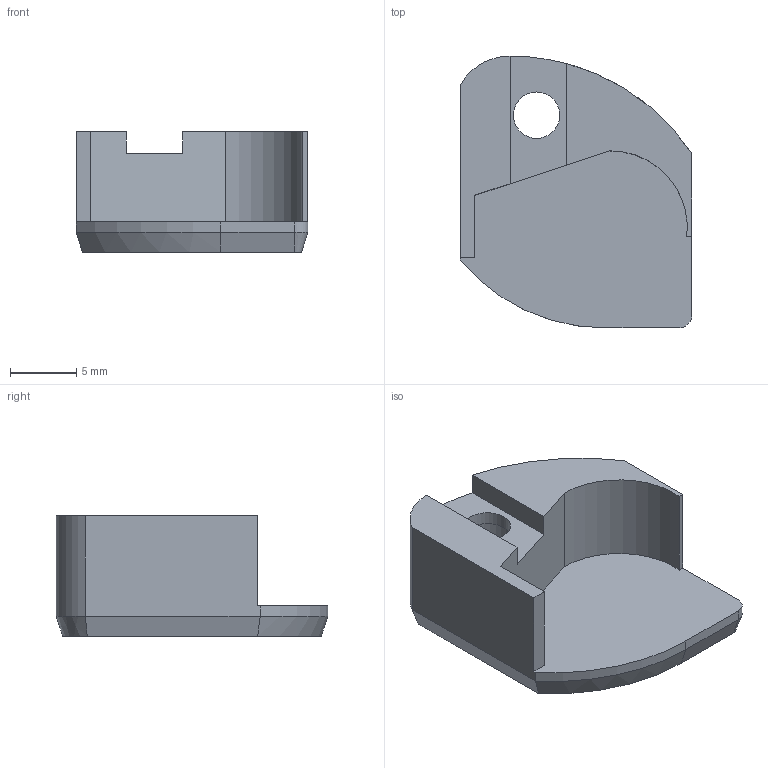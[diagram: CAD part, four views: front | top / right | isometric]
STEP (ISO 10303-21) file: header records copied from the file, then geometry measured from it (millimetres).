
FILE_DESCRIPTION(/* description */ (''),/* implementation_level */ '2;1');
FILE_NAME(/* name */ 'thumb tab side 2 v1.step',/* time_stamp */ '2022-02-13T17:47:28-06:00',/* author */ (''),/* organization */ (''),/* preprocessor_version */ 'ST-DEVELOPER v18.1',/* originating_system */ 'Autodesk Translation Framework v10.13.0.1454',/* authorisation */ '');
FILE_SCHEMA (('AUTOMOTIVE_DESIGN { 1 0 10303 214 3 1 1 }'));
Length unit declared in the file: millimetre
Products named in the file (1): thumb tab side 2
Bounding box: 17.5 x 20.5 x 9.1 mm (x, y, z)
Volume: 1359.4 mm3; surface area: 1299.2 mm2
Topology: 1 solids, 1 shells, 31 faces, 75 edges, 47 vertices
Faces by surface type: plane 19, cylinder 7, cone 5
Full cylindrical faces by diameter (mm): 3.5 x1, 5 x1
Entity records: 937 total; most frequent: CARTESIAN_POINT 163, DIRECTION 156, ORIENTED_EDGE 150, EDGE_CURVE 75, LINE 52, VECTOR 52, AXIS2_PLACEMENT_3D 52, VERTEX_POINT 47
